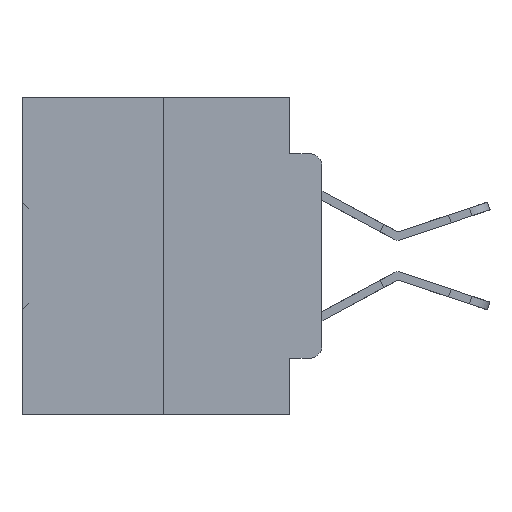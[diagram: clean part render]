
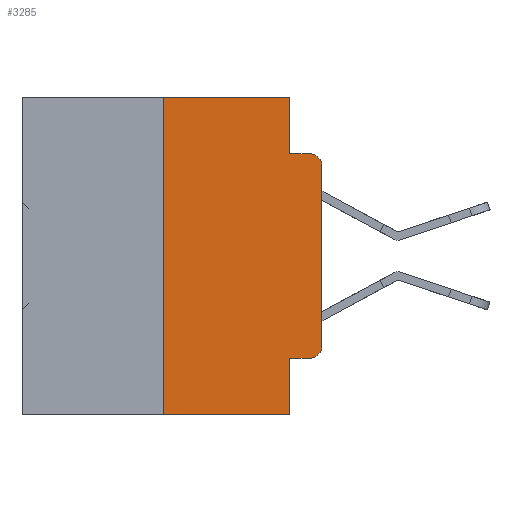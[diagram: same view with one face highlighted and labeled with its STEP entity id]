
A CAD part, left-side view. The second image highlights one B-rep face of the part: STEP entity #3285.
In plain terms, the highlighted planar face has unit normal (-1, 0, 0).
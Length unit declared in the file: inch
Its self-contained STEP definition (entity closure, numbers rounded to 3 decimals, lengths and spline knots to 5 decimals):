
#484 = DIRECTION ( 'NONE',  ( 0., 0., 1. ) ) ;
#610 = CARTESIAN_POINT ( 'NONE',  ( 0., 0.051, -0.0885 ) ) ;
#712 = DIRECTION ( 'NONE',  ( 0., 0., -1. ) ) ;
#1625 = VECTOR ( 'NONE', #12243, 39.37008 ) ;
#1955 = LINE ( 'NONE', #13663, #12041 ) ;
#2117 = FACE_OUTER_BOUND ( 'NONE', #21885, .T. ) ;
#2471 = LINE ( 'NONE', #20151, #1625 ) ;
#2595 = AXIS2_PLACEMENT_3D ( 'NONE', #14878, #23688, #20837 ) ;
#2857 = LINE ( 'NONE', #32017, #33006 ) ;
#3233 = CARTESIAN_POINT ( 'NONE',  ( 0., 0., -0.3915 ) ) ;
#3285 = ADVANCED_FACE ( 'NONE', ( #2117 ), #13442, .F. ) ;
#5118 = VERTEX_POINT ( 'NONE', #26613 ) ;
#5180 = VECTOR ( 'NONE', #31758, 39.37008 ) ;
#5614 = EDGE_CURVE ( 'NONE', #13979, #35777, #8736, .T. ) ;
#6060 = DIRECTION ( 'NONE',  ( 0., -1., 0. ) ) ;
#6081 = ORIENTED_EDGE ( 'NONE', *, *, #25435, .F. ) ;
#6469 = DIRECTION ( 'NONE',  ( -1., 0., 0. ) ) ;
#6601 = ORIENTED_EDGE ( 'NONE', *, *, #12718, .F. ) ;
#7683 = DIRECTION ( 'NONE',  ( 0., 0., -1. ) ) ;
#8237 = EDGE_CURVE ( 'NONE', #26802, #21441, #2857, .T. ) ;
#8364 = CARTESIAN_POINT ( 'NONE',  ( 0., 0.051, 0. ) ) ;
#8473 = AXIS2_PLACEMENT_3D ( 'NONE', #13642, #13822, #7683 ) ;
#8493 = VECTOR ( 'NONE', #35445, 39.37008 ) ;
#8736 = CIRCLE ( 'NONE', #2595, 0.02 ) ;
#8791 = LINE ( 'NONE', #11850, #8493 ) ;
#8939 = LINE ( 'NONE', #32332, #13020 ) ;
#9927 = ORIENTED_EDGE ( 'NONE', *, *, #12747, .T. ) ;
#10324 = AXIS2_PLACEMENT_3D ( 'NONE', #37749, #6469, #712 ) ;
#11133 = CARTESIAN_POINT ( 'NONE',  ( 0., 0.25, 0. ) ) ;
#11479 = CARTESIAN_POINT ( 'NONE',  ( 0., 0., -0.1085 ) ) ;
#11687 = CARTESIAN_POINT ( 'NONE',  ( 0., 0.02, -0.0885 ) ) ;
#11850 = CARTESIAN_POINT ( 'NONE',  ( 0., 0.473, 0. ) ) ;
#12041 = VECTOR ( 'NONE', #28990, 39.37008 ) ;
#12243 = DIRECTION ( 'NONE',  ( 0., 0., 1. ) ) ;
#12718 = EDGE_CURVE ( 'NONE', #24206, #26240, #8791, .T. ) ;
#12747 = EDGE_CURVE ( 'NONE', #26993, #29671, #36058, .T. ) ;
#12980 = CARTESIAN_POINT ( 'NONE',  ( 0., 0., 0. ) ) ;
#13020 = VECTOR ( 'NONE', #6060, 39.37008 ) ;
#13442 = PLANE ( 'NONE',  #8473 ) ;
#13642 = CARTESIAN_POINT ( 'NONE',  ( 0., 0.473, 0. ) ) ;
#13663 = CARTESIAN_POINT ( 'NONE',  ( 0., 0.051, 0. ) ) ;
#13822 = DIRECTION ( 'NONE',  ( 1., 0., 0. ) ) ;
#13954 = EDGE_CURVE ( 'NONE', #26802, #24206, #2471, .T. ) ;
#13979 = VERTEX_POINT ( 'NONE', #11479 ) ;
#14878 = CARTESIAN_POINT ( 'NONE',  ( 0., 0.02, -0.1085 ) ) ;
#16119 = EDGE_CURVE ( 'NONE', #26240, #24710, #1955, .T. ) ;
#16864 = VECTOR ( 'NONE', #484, 39.37008 ) ;
#19661 = ORIENTED_EDGE ( 'NONE', *, *, #32865, .T. ) ;
#20110 = DIRECTION ( 'NONE',  ( 0., -1., 0. ) ) ;
#20151 = CARTESIAN_POINT ( 'NONE',  ( 0., 0.25, 0. ) ) ;
#20720 = DIRECTION ( 'NONE',  ( 0., -1., 0. ) ) ;
#20837 = DIRECTION ( 'NONE',  ( 0., 0., -1. ) ) ;
#21441 = VERTEX_POINT ( 'NONE', #34842 ) ;
#21885 = EDGE_LOOP ( 'NONE', ( #29164, #35854, #22273, #33154, #6601, #36260, #34485, #6081, #19661, #9927 ) ) ;
#21950 = CARTESIAN_POINT ( 'NONE',  ( 0., 0.051, 0. ) ) ;
#22273 = ORIENTED_EDGE ( 'NONE', *, *, #22865, .F. ) ;
#22865 = EDGE_CURVE ( 'NONE', #24710, #35777, #8939, .T. ) ;
#23535 = CARTESIAN_POINT ( 'NONE',  ( 0., 0.051, -0.4115 ) ) ;
#23688 = DIRECTION ( 'NONE',  ( -1., 0., 0. ) ) ;
#24206 = VERTEX_POINT ( 'NONE', #11133 ) ;
#24293 = LINE ( 'NONE', #12980, #16864 ) ;
#24710 = VERTEX_POINT ( 'NONE', #610 ) ;
#25103 = CARTESIAN_POINT ( 'NONE',  ( 0., 0.02, -0.4115 ) ) ;
#25435 = EDGE_CURVE ( 'NONE', #5118, #21441, #37535, .T. ) ;
#25908 = CARTESIAN_POINT ( 'NONE',  ( 0., 0.25, -0.5 ) ) ;
#26240 = VERTEX_POINT ( 'NONE', #21950 ) ;
#26613 = CARTESIAN_POINT ( 'NONE',  ( 0., 0.051, -0.4115 ) ) ;
#26802 = VERTEX_POINT ( 'NONE', #25908 ) ;
#26993 = VERTEX_POINT ( 'NONE', #25103 ) ;
#28990 = DIRECTION ( 'NONE',  ( 0., 0., -1. ) ) ;
#29164 = ORIENTED_EDGE ( 'NONE', *, *, #34377, .T. ) ;
#29671 = VERTEX_POINT ( 'NONE', #3233 ) ;
#31758 = DIRECTION ( 'NONE',  ( 0., 0., -1. ) ) ;
#32017 = CARTESIAN_POINT ( 'NONE',  ( 0., 0.473, -0.5 ) ) ;
#32332 = CARTESIAN_POINT ( 'NONE',  ( 0., 0.051, -0.0885 ) ) ;
#32334 = LINE ( 'NONE', #23535, #34541 ) ;
#32865 = EDGE_CURVE ( 'NONE', #5118, #26993, #32334, .T. ) ;
#33006 = VECTOR ( 'NONE', #20720, 39.37008 ) ;
#33154 = ORIENTED_EDGE ( 'NONE', *, *, #16119, .F. ) ;
#34377 = EDGE_CURVE ( 'NONE', #29671, #13979, #24293, .T. ) ;
#34485 = ORIENTED_EDGE ( 'NONE', *, *, #8237, .T. ) ;
#34541 = VECTOR ( 'NONE', #20110, 39.37008 ) ;
#34842 = CARTESIAN_POINT ( 'NONE',  ( 0., 0.051, -0.5 ) ) ;
#35445 = DIRECTION ( 'NONE',  ( 0., -1., 0. ) ) ;
#35777 = VERTEX_POINT ( 'NONE', #11687 ) ;
#35854 = ORIENTED_EDGE ( 'NONE', *, *, #5614, .T. ) ;
#36058 = CIRCLE ( 'NONE', #10324, 0.02 ) ;
#36260 = ORIENTED_EDGE ( 'NONE', *, *, #13954, .F. ) ;
#37535 = LINE ( 'NONE', #8364, #5180 ) ;
#37749 = CARTESIAN_POINT ( 'NONE',  ( 0., 0.02, -0.3915 ) ) ;
